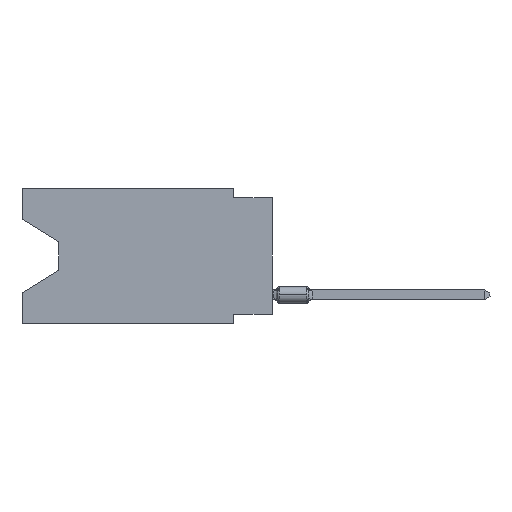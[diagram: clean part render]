
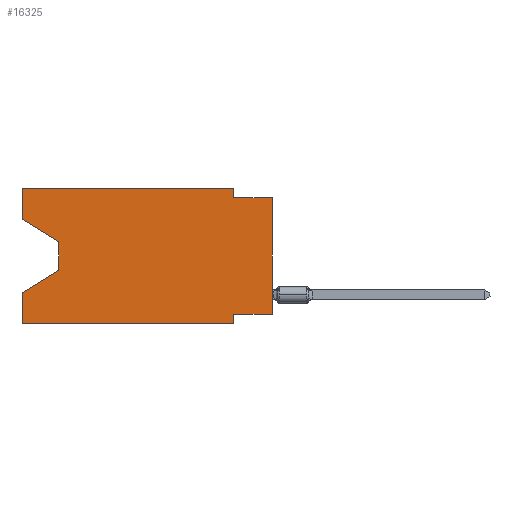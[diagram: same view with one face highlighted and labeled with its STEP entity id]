
A CAD part, left-side view. The second image highlights one B-rep face of the part: STEP entity #16325.
In plain terms, the highlighted planar face has unit normal (-1, 0, 0).
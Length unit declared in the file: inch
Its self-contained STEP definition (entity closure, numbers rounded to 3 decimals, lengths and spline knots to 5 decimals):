
#40 = EDGE_CURVE ( 'NONE', #10930, #18679, #2258, .T. ) ;
#349 = VERTEX_POINT ( 'NONE', #9562 ) ;
#955 = CARTESIAN_POINT ( 'NONE',  ( 0., 0.645, -0.08025 ) ) ;
#1050 = FACE_OUTER_BOUND ( 'NONE', #18940, .T. ) ;
#1156 = CARTESIAN_POINT ( 'NONE',  ( 0., 0., 0. ) ) ;
#1604 = CARTESIAN_POINT ( 'NONE',  ( 0., 0.55, -0.212 ) ) ;
#1621 = EDGE_CURVE ( 'NONE', #8301, #18679, #14576, .T. ) ;
#1769 = LINE ( 'NONE', #4798, #3095 ) ;
#2246 = CARTESIAN_POINT ( 'NONE',  ( 0., 0.1, -0.325 ) ) ;
#2248 = VECTOR ( 'NONE', #12188, 39.37008 ) ;
#2258 = LINE ( 'NONE', #5085, #3716 ) ;
#2406 = CARTESIAN_POINT ( 'NONE',  ( 0., 0., -0.025 ) ) ;
#2411 = DIRECTION ( 'NONE',  ( 0., 0., 1. ) ) ;
#2416 = LINE ( 'NONE', #3916, #2628 ) ;
#2487 = VERTEX_POINT ( 'NONE', #1604 ) ;
#2628 = VECTOR ( 'NONE', #8975, 39.37008 ) ;
#2938 = ORIENTED_EDGE ( 'NONE', *, *, #9571, .T. ) ;
#3095 = VECTOR ( 'NONE', #9727, 39.37008 ) ;
#3508 = EDGE_CURVE ( 'NONE', #2487, #9407, #11746, .T. ) ;
#3599 = ORIENTED_EDGE ( 'NONE', *, *, #40, .F. ) ;
#3716 = VECTOR ( 'NONE', #11823, 39.37008 ) ;
#3916 = CARTESIAN_POINT ( 'NONE',  ( 0., 0.645, 0. ) ) ;
#3981 = CARTESIAN_POINT ( 'NONE',  ( 0., 0.1, -0.35 ) ) ;
#4030 = LINE ( 'NONE', #9196, #2248 ) ;
#4066 = EDGE_CURVE ( 'NONE', #18957, #20626, #4497, .T. ) ;
#4497 = LINE ( 'NONE', #1156, #19462 ) ;
#4597 = DIRECTION ( 'NONE',  ( 0., -1., 0. ) ) ;
#4709 = EDGE_CURVE ( 'NONE', #18957, #10930, #14533, .T. ) ;
#4798 = CARTESIAN_POINT ( 'NONE',  ( 0., 0.1, 0. ) ) ;
#5048 = VECTOR ( 'NONE', #4597, 39.37008 ) ;
#5085 = CARTESIAN_POINT ( 'NONE',  ( 0., 0.1, -0.35 ) ) ;
#5089 = ORIENTED_EDGE ( 'NONE', *, *, #3508, .T. ) ;
#5720 = DIRECTION ( 'NONE',  ( 0., 0., -1. ) ) ;
#6082 = EDGE_CURVE ( 'NONE', #20473, #14776, #1769, .T. ) ;
#6138 = DIRECTION ( 'NONE',  ( 0., -1., 0. ) ) ;
#6273 = DIRECTION ( 'NONE',  ( 0., 1., 0. ) ) ;
#6654 = CARTESIAN_POINT ( 'NONE',  ( 0., 0.645, -0.08025 ) ) ;
#7220 = VECTOR ( 'NONE', #6273, 39.37008 ) ;
#7341 = VECTOR ( 'NONE', #2411, 39.37008 ) ;
#7976 = EDGE_CURVE ( 'NONE', #349, #20473, #10970, .T. ) ;
#8138 = ORIENTED_EDGE ( 'NONE', *, *, #1621, .T. ) ;
#8254 = CARTESIAN_POINT ( 'NONE',  ( 0., 0., -0.325 ) ) ;
#8301 = VERTEX_POINT ( 'NONE', #16056 ) ;
#8975 = DIRECTION ( 'NONE',  ( 0., 0., 1. ) ) ;
#9074 = ORIENTED_EDGE ( 'NONE', *, *, #6082, .F. ) ;
#9124 = LINE ( 'NONE', #955, #19623 ) ;
#9196 = CARTESIAN_POINT ( 'NONE',  ( 0., 0., -0.025 ) ) ;
#9407 = VERTEX_POINT ( 'NONE', #10222 ) ;
#9562 = CARTESIAN_POINT ( 'NONE',  ( 0., 0.645, 0. ) ) ;
#9571 = EDGE_CURVE ( 'NONE', #20948, #2487, #20408, .T. ) ;
#9727 = DIRECTION ( 'NONE',  ( 0., 0., -1. ) ) ;
#9796 = ORIENTED_EDGE ( 'NONE', *, *, #15791, .F. ) ;
#9927 = EDGE_CURVE ( 'NONE', #11213, #20948, #9124, .T. ) ;
#10030 = CARTESIAN_POINT ( 'NONE',  ( 0., 0.55, -0.212 ) ) ;
#10222 = CARTESIAN_POINT ( 'NONE',  ( 0., 0.645, -0.26975 ) ) ;
#10930 = VERTEX_POINT ( 'NONE', #2246 ) ;
#10939 = DIRECTION ( 'NONE',  ( 1., 0., 0. ) ) ;
#10970 = LINE ( 'NONE', #13982, #12767 ) ;
#11044 = DIRECTION ( 'NONE',  ( 0., 0., 1. ) ) ;
#11213 = VERTEX_POINT ( 'NONE', #6654 ) ;
#11251 = CARTESIAN_POINT ( 'NONE',  ( 0., 0.645, -0.35 ) ) ;
#11741 = CARTESIAN_POINT ( 'NONE',  ( 0., 0.55, -0.138 ) ) ;
#11746 = LINE ( 'NONE', #10030, #17639 ) ;
#11823 = DIRECTION ( 'NONE',  ( 0., 0., -1. ) ) ;
#11865 = EDGE_CURVE ( 'NONE', #8301, #9407, #17110, .T. ) ;
#12188 = DIRECTION ( 'NONE',  ( 0., -1., 0. ) ) ;
#12532 = ORIENTED_EDGE ( 'NONE', *, *, #9927, .T. ) ;
#12573 = ORIENTED_EDGE ( 'NONE', *, *, #4066, .T. ) ;
#12766 = VECTOR ( 'NONE', #5720, 39.37008 ) ;
#12767 = VECTOR ( 'NONE', #6138, 39.37008 ) ;
#13461 = CARTESIAN_POINT ( 'NONE',  ( 0., 0.1, -0.025 ) ) ;
#13476 = CARTESIAN_POINT ( 'NONE',  ( 0., 0.1, 0. ) ) ;
#13982 = CARTESIAN_POINT ( 'NONE',  ( 0., 0.645, 0. ) ) ;
#14487 = EDGE_CURVE ( 'NONE', #11213, #349, #2416, .T. ) ;
#14533 = LINE ( 'NONE', #21060, #7220 ) ;
#14576 = LINE ( 'NONE', #11251, #5048 ) ;
#14776 = VERTEX_POINT ( 'NONE', #13461 ) ;
#15555 = DIRECTION ( 'NONE',  ( 0., -0.855, -0.519 ) ) ;
#15791 = EDGE_CURVE ( 'NONE', #14776, #20626, #4030, .T. ) ;
#16056 = CARTESIAN_POINT ( 'NONE',  ( 0., 0.645, -0.35 ) ) ;
#16325 = ADVANCED_FACE ( 'NONE', ( #1050 ), #20903, .F. ) ;
#17110 = LINE ( 'NONE', #18613, #7341 ) ;
#17258 = DIRECTION ( 'NONE',  ( 0., 0., -1. ) ) ;
#17367 = CARTESIAN_POINT ( 'NONE',  ( 0., 0.645, 0. ) ) ;
#17639 = VECTOR ( 'NONE', #18277, 39.37008 ) ;
#18277 = DIRECTION ( 'NONE',  ( 0., 0.855, -0.519 ) ) ;
#18613 = CARTESIAN_POINT ( 'NONE',  ( 0., 0.645, 0. ) ) ;
#18679 = VERTEX_POINT ( 'NONE', #3981 ) ;
#18940 = EDGE_LOOP ( 'NONE', ( #12532, #2938, #5089, #20235, #8138, #3599, #19192, #12573, #9796, #9074, #21206, #20719 ) ) ;
#18957 = VERTEX_POINT ( 'NONE', #8254 ) ;
#19118 = CARTESIAN_POINT ( 'NONE',  ( 0., 0.55, -0.138 ) ) ;
#19192 = ORIENTED_EDGE ( 'NONE', *, *, #4709, .F. ) ;
#19414 = AXIS2_PLACEMENT_3D ( 'NONE', #17367, #10939, #17258 ) ;
#19462 = VECTOR ( 'NONE', #11044, 39.37008 ) ;
#19623 = VECTOR ( 'NONE', #15555, 39.37008 ) ;
#20235 = ORIENTED_EDGE ( 'NONE', *, *, #11865, .F. ) ;
#20408 = LINE ( 'NONE', #19118, #12766 ) ;
#20473 = VERTEX_POINT ( 'NONE', #13476 ) ;
#20626 = VERTEX_POINT ( 'NONE', #2406 ) ;
#20719 = ORIENTED_EDGE ( 'NONE', *, *, #14487, .F. ) ;
#20903 = PLANE ( 'NONE',  #19414 ) ;
#20948 = VERTEX_POINT ( 'NONE', #11741 ) ;
#21060 = CARTESIAN_POINT ( 'NONE',  ( 0., 0., -0.325 ) ) ;
#21206 = ORIENTED_EDGE ( 'NONE', *, *, #7976, .F. ) ;
